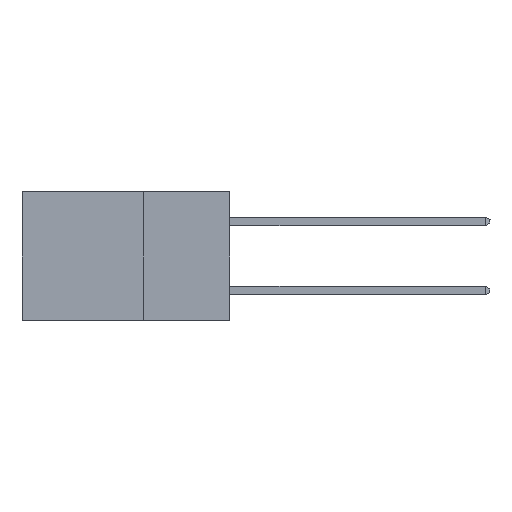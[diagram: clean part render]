
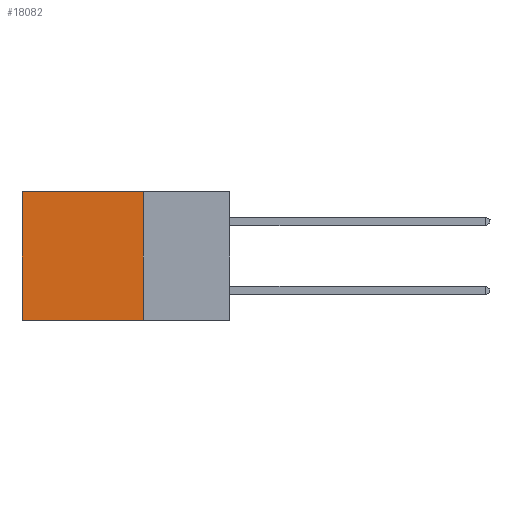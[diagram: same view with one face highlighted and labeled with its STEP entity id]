
A CAD part, left-side view. The second image highlights one B-rep face of the part: STEP entity #18082.
In plain terms, the highlighted planar face has unit normal (-1, 0, 0).
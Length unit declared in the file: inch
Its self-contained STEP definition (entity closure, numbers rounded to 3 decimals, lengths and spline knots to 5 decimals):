
#2604 = LINE ( 'NONE', #21597, #17496 ) ;
#2615 = CARTESIAN_POINT ( 'NONE',  ( 0.2615, 0.25, -0.37 ) ) ;
#2834 = ORIENTED_EDGE ( 'NONE', *, *, #4195, .F. ) ;
#3143 = CARTESIAN_POINT ( 'NONE',  ( 0.2615, 0.25, -0.37 ) ) ;
#4087 = VECTOR ( 'NONE', #21478, 39.37008 ) ;
#4195 = EDGE_CURVE ( 'NONE', #13416, #23796, #15923, .T. ) ;
#4366 = VERTEX_POINT ( 'NONE', #18316 ) ;
#5107 = ORIENTED_EDGE ( 'NONE', *, *, #22817, .T. ) ;
#5313 = LINE ( 'NONE', #18875, #16877 ) ;
#5509 = DIRECTION ( 'NONE',  ( 1., 0., 0. ) ) ;
#5723 = DIRECTION ( 'NONE',  ( 0., 1., 0. ) ) ;
#6575 = VECTOR ( 'NONE', #5723, 39.37008 ) ;
#7849 = LINE ( 'NONE', #13869, #6575 ) ;
#9028 = FACE_OUTER_BOUND ( 'NONE', #19723, .T. ) ;
#9209 = DIRECTION ( 'NONE',  ( 0., 0., -1. ) ) ;
#9519 = CARTESIAN_POINT ( 'NONE',  ( 0.2615, 0.25, 0. ) ) ;
#9915 = VERTEX_POINT ( 'NONE', #9519 ) ;
#10038 = EDGE_CURVE ( 'NONE', #4366, #23796, #2604, .T. ) ;
#12138 = DIRECTION ( 'NONE',  ( 0., 0., -1. ) ) ;
#12352 = ORIENTED_EDGE ( 'NONE', *, *, #10038, .T. ) ;
#12418 = ORIENTED_EDGE ( 'NONE', *, *, #15837, .F. ) ;
#13416 = VERTEX_POINT ( 'NONE', #23439 ) ;
#13869 = CARTESIAN_POINT ( 'NONE',  ( 0.2615, 0.25, 0. ) ) ;
#14921 = DIRECTION ( 'NONE',  ( 0., 0., -1. ) ) ;
#15837 = EDGE_CURVE ( 'NONE', #9915, #13416, #5313, .T. ) ;
#15923 = LINE ( 'NONE', #2615, #4087 ) ;
#16877 = VECTOR ( 'NONE', #9209, 39.37008 ) ;
#17496 = VECTOR ( 'NONE', #12138, 39.37008 ) ;
#18082 = ADVANCED_FACE ( 'NONE', ( #9028 ), #24735, .F. ) ;
#18307 = CARTESIAN_POINT ( 'NONE',  ( 0.2615, 0.6, -0.37 ) ) ;
#18316 = CARTESIAN_POINT ( 'NONE',  ( 0.2615, 0.6, 0. ) ) ;
#18875 = CARTESIAN_POINT ( 'NONE',  ( 0.2615, 0.25, -0.37 ) ) ;
#19723 = EDGE_LOOP ( 'NONE', ( #12352, #2834, #12418, #5107 ) ) ;
#21478 = DIRECTION ( 'NONE',  ( 0., 1., 0. ) ) ;
#21597 = CARTESIAN_POINT ( 'NONE',  ( 0.2615, 0.6, -0.37 ) ) ;
#22182 = AXIS2_PLACEMENT_3D ( 'NONE', #3143, #5509, #14921 ) ;
#22817 = EDGE_CURVE ( 'NONE', #9915, #4366, #7849, .T. ) ;
#23439 = CARTESIAN_POINT ( 'NONE',  ( 0.2615, 0.25, -0.37 ) ) ;
#23796 = VERTEX_POINT ( 'NONE', #18307 ) ;
#24735 = PLANE ( 'NONE',  #22182 ) ;
